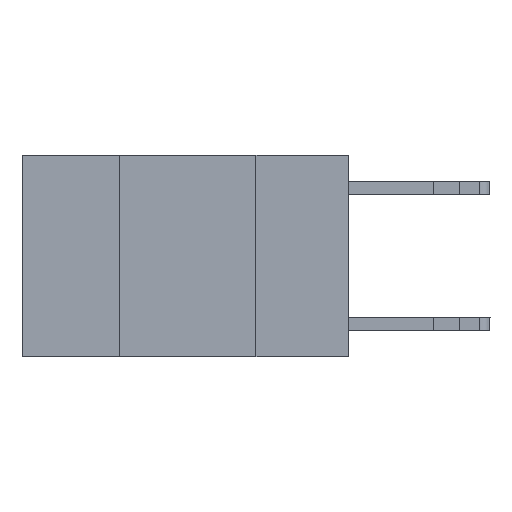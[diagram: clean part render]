
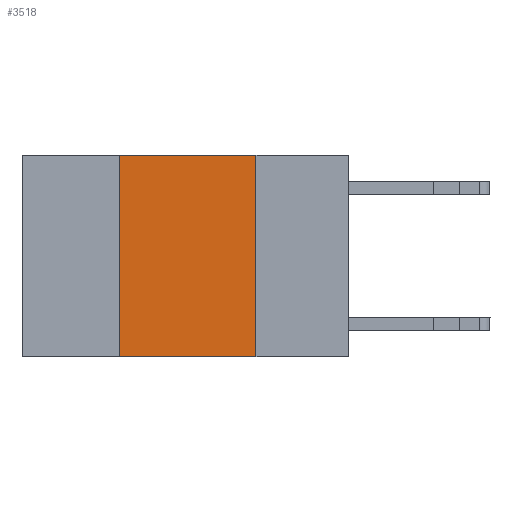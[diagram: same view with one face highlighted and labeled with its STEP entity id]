
A CAD part, left-side view. The second image highlights one B-rep face of the part: STEP entity #3518.
In plain terms, the highlighted planar face has unit normal (-1, 0, 0).
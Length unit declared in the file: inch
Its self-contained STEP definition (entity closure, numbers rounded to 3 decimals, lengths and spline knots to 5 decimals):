
#175 = CARTESIAN_POINT ( 'NONE',  ( 0., 0.17, -0.37 ) ) ;
#824 = EDGE_CURVE ( 'NONE', #21197, #4009, #4251, .T. ) ;
#2280 = VECTOR ( 'NONE', #19563, 39.37008 ) ;
#2871 = VERTEX_POINT ( 'NONE', #16378 ) ;
#3459 = DIRECTION ( 'NONE',  ( 0., 0., 1. ) ) ;
#3518 = ADVANCED_FACE ( 'NONE', ( #12935 ), #8315, .F. ) ;
#3557 = CARTESIAN_POINT ( 'NONE',  ( 0., 0.42, 0. ) ) ;
#3826 = EDGE_CURVE ( 'NONE', #21197, #2871, #11227, .T. ) ;
#3928 = DIRECTION ( 'NONE',  ( 0., 0., -1. ) ) ;
#4009 = VERTEX_POINT ( 'NONE', #175 ) ;
#4026 = CARTESIAN_POINT ( 'NONE',  ( 0., 0.17, 0. ) ) ;
#4251 = LINE ( 'NONE', #5281, #2280 ) ;
#4970 = EDGE_LOOP ( 'NONE', ( #9932, #7996, #25557, #14287 ) ) ;
#5281 = CARTESIAN_POINT ( 'NONE',  ( 0., 0.6, -0.37 ) ) ;
#5768 = VERTEX_POINT ( 'NONE', #15102 ) ;
#7862 = DIRECTION ( 'NONE',  ( 0., 0., -1. ) ) ;
#7891 = DIRECTION ( 'NONE',  ( 1., 0., 0. ) ) ;
#7996 = ORIENTED_EDGE ( 'NONE', *, *, #26223, .F. ) ;
#8016 = CARTESIAN_POINT ( 'NONE',  ( 0., 0.6, 0. ) ) ;
#8315 = PLANE ( 'NONE',  #25552 ) ;
#9662 = EDGE_CURVE ( 'NONE', #5768, #4009, #20089, .T. ) ;
#9932 = ORIENTED_EDGE ( 'NONE', *, *, #9662, .F. ) ;
#10806 = VECTOR ( 'NONE', #3459, 39.37008 ) ;
#11227 = LINE ( 'NONE', #3557, #10806 ) ;
#12370 = DIRECTION ( 'NONE',  ( 0., -1., 0. ) ) ;
#12935 = FACE_OUTER_BOUND ( 'NONE', #4970, .T. ) ;
#13681 = CARTESIAN_POINT ( 'NONE',  ( 0., 0.42, -0.37 ) ) ;
#14287 = ORIENTED_EDGE ( 'NONE', *, *, #824, .T. ) ;
#14498 = CARTESIAN_POINT ( 'NONE',  ( 0., 0.6, 0. ) ) ;
#15102 = CARTESIAN_POINT ( 'NONE',  ( 0., 0.17, 0. ) ) ;
#16378 = CARTESIAN_POINT ( 'NONE',  ( 0., 0.42, 0. ) ) ;
#19563 = DIRECTION ( 'NONE',  ( 0., -1., 0. ) ) ;
#19669 = VECTOR ( 'NONE', #3928, 39.37008 ) ;
#20089 = LINE ( 'NONE', #4026, #19669 ) ;
#21197 = VERTEX_POINT ( 'NONE', #13681 ) ;
#24889 = VECTOR ( 'NONE', #12370, 39.37008 ) ;
#25552 = AXIS2_PLACEMENT_3D ( 'NONE', #8016, #7891, #7862 ) ;
#25557 = ORIENTED_EDGE ( 'NONE', *, *, #3826, .F. ) ;
#25653 = LINE ( 'NONE', #14498, #24889 ) ;
#26223 = EDGE_CURVE ( 'NONE', #2871, #5768, #25653, .T. ) ;
